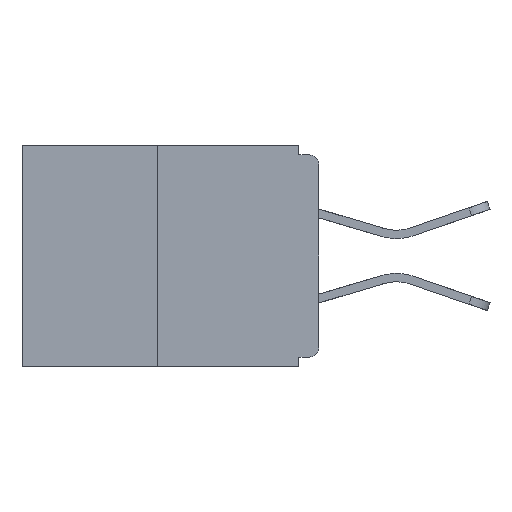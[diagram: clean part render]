
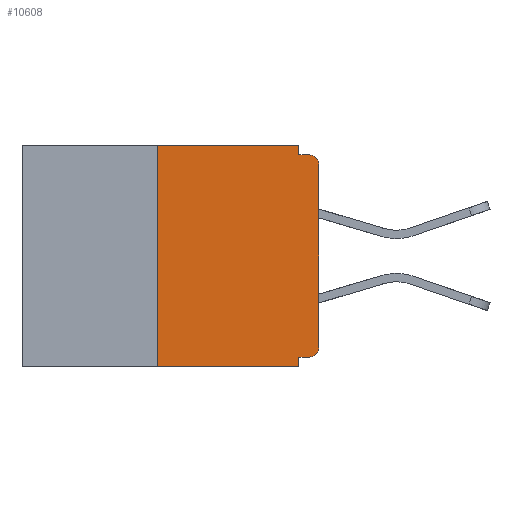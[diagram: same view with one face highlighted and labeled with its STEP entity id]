
A CAD part, left-side view. The second image highlights one B-rep face of the part: STEP entity #10608.
In plain terms, the highlighted planar face has unit normal (-1, 0, 0).
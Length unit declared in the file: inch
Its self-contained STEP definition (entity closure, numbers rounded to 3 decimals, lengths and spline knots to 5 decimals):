
#214 = ORIENTED_EDGE ( 'NONE', *, *, #5742, .F. ) ;
#442 = CARTESIAN_POINT ( 'NONE',  ( 0., 0.25, 0. ) ) ;
#643 = CARTESIAN_POINT ( 'NONE',  ( 0., 0., -0.313 ) ) ;
#765 = ORIENTED_EDGE ( 'NONE', *, *, #5607, .F. ) ;
#960 = VERTEX_POINT ( 'NONE', #1910 ) ;
#1426 = DIRECTION ( 'NONE',  ( 0., 0., -1. ) ) ;
#1494 = EDGE_CURVE ( 'NONE', #3348, #3522, #7399, .T. ) ;
#1530 = VERTEX_POINT ( 'NONE', #11861 ) ;
#1533 = CARTESIAN_POINT ( 'NONE',  ( 0., 0.46, 0. ) ) ;
#1910 = CARTESIAN_POINT ( 'NONE',  ( 0., 0.031, -0.328 ) ) ;
#2062 = VERTEX_POINT ( 'NONE', #10729 ) ;
#2227 = CARTESIAN_POINT ( 'NONE',  ( 0., 0.25, 0. ) ) ;
#2839 = CARTESIAN_POINT ( 'NONE',  ( 0., 0., -0.015 ) ) ;
#3283 = DIRECTION ( 'NONE',  ( -1., 0., 0. ) ) ;
#3348 = VERTEX_POINT ( 'NONE', #8488 ) ;
#3467 = CARTESIAN_POINT ( 'NONE',  ( 0., 0.015, -0.03 ) ) ;
#3522 = VERTEX_POINT ( 'NONE', #13336 ) ;
#3631 = VECTOR ( 'NONE', #13915, 39.37008 ) ;
#3705 = DIRECTION ( 'NONE',  ( 0., 0., -1. ) ) ;
#3765 = CARTESIAN_POINT ( 'NONE',  ( 0., 0.031, -0.343 ) ) ;
#4135 = CIRCLE ( 'NONE', #9303, 0.015 ) ;
#4637 = DIRECTION ( 'NONE',  ( 0., 0., -1. ) ) ;
#4658 = DIRECTION ( 'NONE',  ( 0., -1., 0. ) ) ;
#4693 = EDGE_CURVE ( 'NONE', #13316, #3348, #11547, .T. ) ;
#4861 = EDGE_CURVE ( 'NONE', #12698, #15584, #4135, .T. ) ;
#5092 = FACE_OUTER_BOUND ( 'NONE', #6356, .T. ) ;
#5607 = EDGE_CURVE ( 'NONE', #2062, #13316, #5718, .T. ) ;
#5685 = VERTEX_POINT ( 'NONE', #3765 ) ;
#5718 = LINE ( 'NONE', #442, #18547 ) ;
#5742 = EDGE_CURVE ( 'NONE', #960, #5685, #18083, .T. ) ;
#5879 = VECTOR ( 'NONE', #17136, 39.37008 ) ;
#5970 = ORIENTED_EDGE ( 'NONE', *, *, #4861, .T. ) ;
#6356 = EDGE_LOOP ( 'NONE', ( #13580, #765, #16740, #214, #11525, #5970, #8756, #14970, #13379, #14281 ) ) ;
#6587 = EDGE_CURVE ( 'NONE', #1530, #15077, #16493, .T. ) ;
#7399 = LINE ( 'NONE', #17811, #14111 ) ;
#7446 = EDGE_CURVE ( 'NONE', #15584, #1530, #12620, .T. ) ;
#7789 = DIRECTION ( 'NONE',  ( 0., 0., -1. ) ) ;
#7906 = VECTOR ( 'NONE', #16815, 39.37008 ) ;
#8488 = CARTESIAN_POINT ( 'NONE',  ( 0., 0.031, 0. ) ) ;
#8541 = AXIS2_PLACEMENT_3D ( 'NONE', #1533, #11619, #17388 ) ;
#8696 = CARTESIAN_POINT ( 'NONE',  ( 0., 0., -0.328 ) ) ;
#8756 = ORIENTED_EDGE ( 'NONE', *, *, #7446, .T. ) ;
#9134 = VECTOR ( 'NONE', #13020, 39.37008 ) ;
#9206 = CARTESIAN_POINT ( 'NONE',  ( 0., 0.015, -0.015 ) ) ;
#9303 = AXIS2_PLACEMENT_3D ( 'NONE', #12852, #14315, #1426 ) ;
#10545 = EDGE_CURVE ( 'NONE', #3522, #15077, #10720, .T. ) ;
#10608 = ADVANCED_FACE ( 'NONE', ( #5092 ), #12718, .F. ) ;
#10720 = LINE ( 'NONE', #2839, #9134 ) ;
#10729 = CARTESIAN_POINT ( 'NONE',  ( 0., 0.25, -0.343 ) ) ;
#10939 = CARTESIAN_POINT ( 'NONE',  ( 0., 0., 0. ) ) ;
#11525 = ORIENTED_EDGE ( 'NONE', *, *, #13567, .F. ) ;
#11547 = LINE ( 'NONE', #14619, #18080 ) ;
#11619 = DIRECTION ( 'NONE',  ( 1., 0., 0. ) ) ;
#11861 = CARTESIAN_POINT ( 'NONE',  ( 0., 0., -0.03 ) ) ;
#12252 = CARTESIAN_POINT ( 'NONE',  ( 0., 0.031, -0.343 ) ) ;
#12559 = CARTESIAN_POINT ( 'NONE',  ( 0., 0.015, -0.328 ) ) ;
#12620 = LINE ( 'NONE', #10939, #7906 ) ;
#12698 = VERTEX_POINT ( 'NONE', #12559 ) ;
#12718 = PLANE ( 'NONE',  #8541 ) ;
#12818 = LINE ( 'NONE', #14824, #3631 ) ;
#12852 = CARTESIAN_POINT ( 'NONE',  ( 0., 0.015, -0.313 ) ) ;
#13020 = DIRECTION ( 'NONE',  ( 0., -1., 0. ) ) ;
#13187 = EDGE_CURVE ( 'NONE', #2062, #5685, #12818, .T. ) ;
#13316 = VERTEX_POINT ( 'NONE', #2227 ) ;
#13336 = CARTESIAN_POINT ( 'NONE',  ( 0., 0.031, -0.015 ) ) ;
#13365 = DIRECTION ( 'NONE',  ( 0., 0., 1. ) ) ;
#13379 = ORIENTED_EDGE ( 'NONE', *, *, #10545, .F. ) ;
#13567 = EDGE_CURVE ( 'NONE', #12698, #960, #15072, .T. ) ;
#13580 = ORIENTED_EDGE ( 'NONE', *, *, #4693, .F. ) ;
#13915 = DIRECTION ( 'NONE',  ( 0., -1., 0. ) ) ;
#14111 = VECTOR ( 'NONE', #4637, 39.37008 ) ;
#14281 = ORIENTED_EDGE ( 'NONE', *, *, #1494, .F. ) ;
#14315 = DIRECTION ( 'NONE',  ( -1., 0., 0. ) ) ;
#14619 = CARTESIAN_POINT ( 'NONE',  ( 0., 0.46, 0. ) ) ;
#14824 = CARTESIAN_POINT ( 'NONE',  ( 0., 0.46, -0.343 ) ) ;
#14970 = ORIENTED_EDGE ( 'NONE', *, *, #6587, .T. ) ;
#15072 = LINE ( 'NONE', #8696, #5879 ) ;
#15077 = VERTEX_POINT ( 'NONE', #9206 ) ;
#15375 = VECTOR ( 'NONE', #3705, 39.37008 ) ;
#15584 = VERTEX_POINT ( 'NONE', #643 ) ;
#16493 = CIRCLE ( 'NONE', #16806, 0.015 ) ;
#16740 = ORIENTED_EDGE ( 'NONE', *, *, #13187, .T. ) ;
#16806 = AXIS2_PLACEMENT_3D ( 'NONE', #3467, #3283, #7789 ) ;
#16815 = DIRECTION ( 'NONE',  ( 0., 0., 1. ) ) ;
#17136 = DIRECTION ( 'NONE',  ( 0., 1., 0. ) ) ;
#17388 = DIRECTION ( 'NONE',  ( 0., 0., -1. ) ) ;
#17811 = CARTESIAN_POINT ( 'NONE',  ( 0., 0.031, 0. ) ) ;
#18080 = VECTOR ( 'NONE', #4658, 39.37008 ) ;
#18083 = LINE ( 'NONE', #12252, #15375 ) ;
#18547 = VECTOR ( 'NONE', #13365, 39.37008 ) ;
